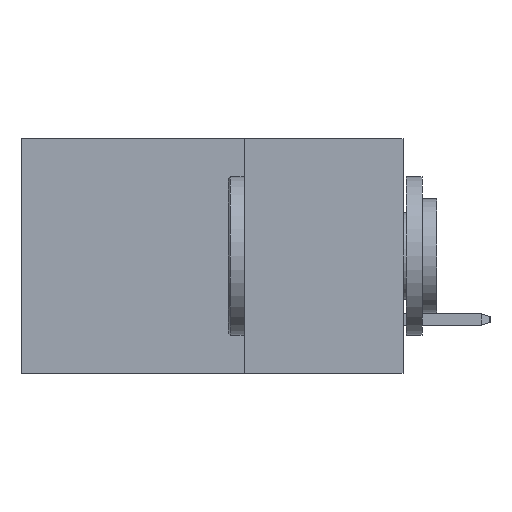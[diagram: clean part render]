
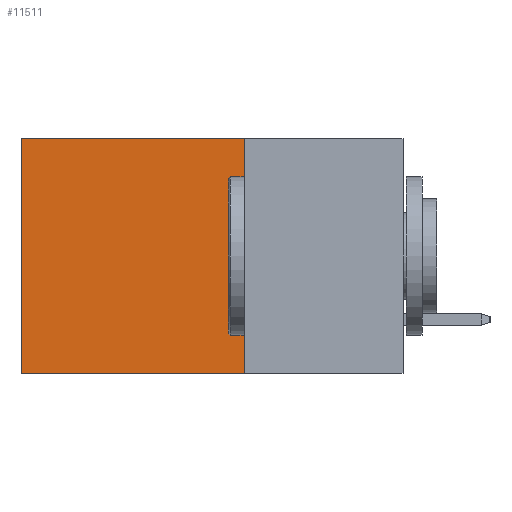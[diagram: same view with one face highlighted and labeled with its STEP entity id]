
A CAD part, left-side view. The second image highlights one B-rep face of the part: STEP entity #11511.
In plain terms, the highlighted planar face has unit normal (-1, 0, 0).
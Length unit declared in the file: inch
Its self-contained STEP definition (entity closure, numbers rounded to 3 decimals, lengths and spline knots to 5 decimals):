
#47 = VECTOR ( 'NONE', #9760, 39.37008 ) ;
#352 = EDGE_CURVE ( 'NONE', #8307, #2932, #6777, .T. ) ;
#578 = LINE ( 'NONE', #9812, #5680 ) ;
#1219 = EDGE_CURVE ( 'NONE', #2932, #3682, #11688, .T. ) ;
#1495 = ORIENTED_EDGE ( 'NONE', *, *, #11966, .F. ) ;
#2192 = AXIS2_PLACEMENT_3D ( 'NONE', #5746, #5474, #7558 ) ;
#2343 = ORIENTED_EDGE ( 'NONE', *, *, #2912, .F. ) ;
#2912 = EDGE_CURVE ( 'NONE', #6333, #3682, #578, .T. ) ;
#2932 = VERTEX_POINT ( 'NONE', #4661 ) ;
#3682 = VERTEX_POINT ( 'NONE', #3761 ) ;
#3761 = CARTESIAN_POINT ( 'NONE',  ( 0.2875, 0.6, -0.37 ) ) ;
#4305 = EDGE_LOOP ( 'NONE', ( #9222, #2343, #1495, #11161 ) ) ;
#4661 = CARTESIAN_POINT ( 'NONE',  ( 0.2875, 0.6, 0. ) ) ;
#4714 = CARTESIAN_POINT ( 'NONE',  ( 0.2875, 0.25, 0. ) ) ;
#5287 = CARTESIAN_POINT ( 'NONE',  ( 0.2875, 0.25, 0. ) ) ;
#5474 = DIRECTION ( 'NONE',  ( 1., 0., 0. ) ) ;
#5597 = LINE ( 'NONE', #12753, #47 ) ;
#5680 = VECTOR ( 'NONE', #8873, 39.37008 ) ;
#5746 = CARTESIAN_POINT ( 'NONE',  ( 0.2875, 0.25, 0. ) ) ;
#6333 = VERTEX_POINT ( 'NONE', #11144 ) ;
#6752 = PLANE ( 'NONE',  #2192 ) ;
#6777 = LINE ( 'NONE', #4714, #11830 ) ;
#6844 = DIRECTION ( 'NONE',  ( 0., 1., 0. ) ) ;
#7558 = DIRECTION ( 'NONE',  ( 0., 0., -1. ) ) ;
#7752 = FACE_OUTER_BOUND ( 'NONE', #4305, .T. ) ;
#7896 = VECTOR ( 'NONE', #10701, 39.37008 ) ;
#8307 = VERTEX_POINT ( 'NONE', #5287 ) ;
#8873 = DIRECTION ( 'NONE',  ( 0., 1., 0. ) ) ;
#9222 = ORIENTED_EDGE ( 'NONE', *, *, #1219, .T. ) ;
#9760 = DIRECTION ( 'NONE',  ( 0., 0., -1. ) ) ;
#9812 = CARTESIAN_POINT ( 'NONE',  ( 0.2875, 0.25, -0.37 ) ) ;
#9826 = CARTESIAN_POINT ( 'NONE',  ( 0.2875, 0.6, 0. ) ) ;
#10701 = DIRECTION ( 'NONE',  ( 0., 0., -1. ) ) ;
#11144 = CARTESIAN_POINT ( 'NONE',  ( 0.2875, 0.25, -0.37 ) ) ;
#11161 = ORIENTED_EDGE ( 'NONE', *, *, #352, .T. ) ;
#11511 = ADVANCED_FACE ( 'NONE', ( #7752 ), #6752, .F. ) ;
#11688 = LINE ( 'NONE', #9826, #7896 ) ;
#11830 = VECTOR ( 'NONE', #6844, 39.37008 ) ;
#11966 = EDGE_CURVE ( 'NONE', #8307, #6333, #5597, .T. ) ;
#12753 = CARTESIAN_POINT ( 'NONE',  ( 0.2875, 0.25, 0. ) ) ;
